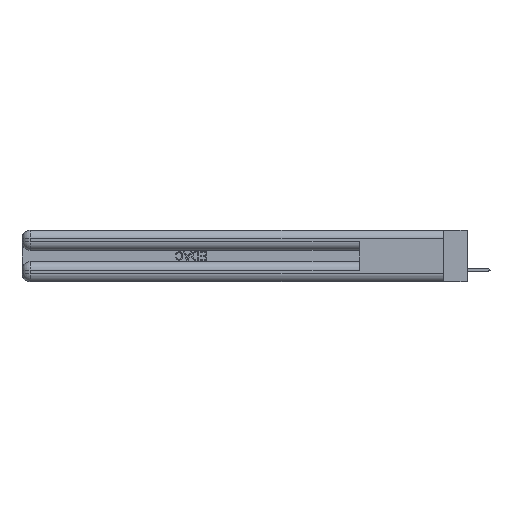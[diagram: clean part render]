
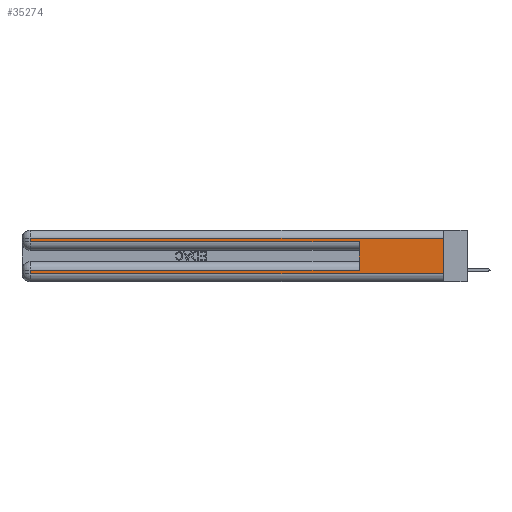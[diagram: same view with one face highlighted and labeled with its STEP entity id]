
A CAD part, left-side view. The second image highlights one B-rep face of the part: STEP entity #35274.
In plain terms, the highlighted planar face has unit normal (-1, 0, 0).
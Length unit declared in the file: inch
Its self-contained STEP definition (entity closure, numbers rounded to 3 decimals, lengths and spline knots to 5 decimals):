
#244 = AXIS2_PLACEMENT_3D ( 'NONE', #25660, #37172, #13451 ) ;
#273 = VECTOR ( 'NONE', #11970, 39.37008 ) ;
#737 = VECTOR ( 'NONE', #44682, 39.37008 ) ;
#2369 = ORIENTED_EDGE ( 'NONE', *, *, #52195, .F. ) ;
#2688 = CARTESIAN_POINT ( 'NONE',  ( 0., 0., 0.06 ) ) ;
#2759 = EDGE_CURVE ( 'NONE', #9822, #37819, #8319, .T. ) ;
#3544 = LINE ( 'NONE', #23982, #273 ) ;
#3567 = ORIENTED_EDGE ( 'NONE', *, *, #43821, .T. ) ;
#4104 = VERTEX_POINT ( 'NONE', #32867 ) ;
#5280 = VECTOR ( 'NONE', #36369, 39.37008 ) ;
#6200 = VERTEX_POINT ( 'NONE', #35007 ) ;
#7194 = DIRECTION ( 'NONE',  ( 0., -1., 0. ) ) ;
#7278 = EDGE_CURVE ( 'NONE', #9822, #4104, #24568, .T. ) ;
#8319 = LINE ( 'NONE', #12839, #49894 ) ;
#9822 = VERTEX_POINT ( 'NONE', #9959 ) ;
#9959 = CARTESIAN_POINT ( 'NONE',  ( 0., 0., 0.31 ) ) ;
#11970 = DIRECTION ( 'NONE',  ( 0., -1., 0. ) ) ;
#12839 = CARTESIAN_POINT ( 'NONE',  ( 0., 0., 0.37 ) ) ;
#13278 = CARTESIAN_POINT ( 'NONE',  ( 0., 2.94, 0.37 ) ) ;
#13451 = DIRECTION ( 'NONE',  ( 0., 0., -1. ) ) ;
#14044 = VERTEX_POINT ( 'NONE', #23625 ) ;
#14071 = EDGE_CURVE ( 'NONE', #27638, #6200, #3544, .T. ) ;
#15268 = EDGE_CURVE ( 'NONE', #44468, #14044, #18999, .T. ) ;
#16174 = CARTESIAN_POINT ( 'NONE',  ( 0., 0.6, 0.145 ) ) ;
#16222 = LINE ( 'NONE', #2688, #24554 ) ;
#18999 = LINE ( 'NONE', #19157, #38222 ) ;
#19157 = CARTESIAN_POINT ( 'NONE',  ( 0., 0., 0.085 ) ) ;
#21005 = DIRECTION ( 'NONE',  ( 0., 0., -1. ) ) ;
#22617 = VECTOR ( 'NONE', #49697, 39.37008 ) ;
#23351 = ORIENTED_EDGE ( 'NONE', *, *, #15268, .T. ) ;
#23366 = VERTEX_POINT ( 'NONE', #47547 ) ;
#23625 = CARTESIAN_POINT ( 'NONE',  ( 0., 2.94, 0.085 ) ) ;
#23982 = CARTESIAN_POINT ( 'NONE',  ( 0., 0., 0.285 ) ) ;
#24554 = VECTOR ( 'NONE', #7194, 39.37008 ) ;
#24568 = LINE ( 'NONE', #24660, #5280 ) ;
#24660 = CARTESIAN_POINT ( 'NONE',  ( 0., 0., 0.31 ) ) ;
#24859 = ORIENTED_EDGE ( 'NONE', *, *, #7278, .T. ) ;
#24878 = CARTESIAN_POINT ( 'NONE',  ( 0., 2.94, 0.37 ) ) ;
#25126 = CARTESIAN_POINT ( 'NONE',  ( 0., 2.94, 0.285 ) ) ;
#25660 = CARTESIAN_POINT ( 'NONE',  ( 0., 0., 0.37 ) ) ;
#26672 = CARTESIAN_POINT ( 'NONE',  ( 0., 0., 0.06 ) ) ;
#26888 = EDGE_CURVE ( 'NONE', #14044, #23366, #27927, .T. ) ;
#27638 = VERTEX_POINT ( 'NONE', #25126 ) ;
#27666 = DIRECTION ( 'NONE',  ( 0., 1., 0. ) ) ;
#27927 = LINE ( 'NONE', #13278, #30411 ) ;
#30411 = VECTOR ( 'NONE', #50302, 39.37008 ) ;
#32867 = CARTESIAN_POINT ( 'NONE',  ( 0., 2.94, 0.31 ) ) ;
#35007 = CARTESIAN_POINT ( 'NONE',  ( 0., 0.6, 0.285 ) ) ;
#35274 = ADVANCED_FACE ( 'NONE', ( #50632 ), #41563, .F. ) ;
#36369 = DIRECTION ( 'NONE',  ( 0., 1., 0. ) ) ;
#37172 = DIRECTION ( 'NONE',  ( 1., 0., 0. ) ) ;
#37363 = LINE ( 'NONE', #16174, #737 ) ;
#37456 = ORIENTED_EDGE ( 'NONE', *, *, #26888, .T. ) ;
#37819 = VERTEX_POINT ( 'NONE', #26672 ) ;
#38222 = VECTOR ( 'NONE', #27666, 39.37008 ) ;
#41563 = PLANE ( 'NONE',  #244 ) ;
#43702 = ORIENTED_EDGE ( 'NONE', *, *, #2759, .F. ) ;
#43821 = EDGE_CURVE ( 'NONE', #4104, #27638, #45172, .T. ) ;
#44468 = VERTEX_POINT ( 'NONE', #48845 ) ;
#44682 = DIRECTION ( 'NONE',  ( 0., 0., 1. ) ) ;
#44870 = ORIENTED_EDGE ( 'NONE', *, *, #14071, .T. ) ;
#45172 = LINE ( 'NONE', #24878, #22617 ) ;
#45265 = EDGE_LOOP ( 'NONE', ( #43702, #24859, #3567, #44870, #2369, #23351, #37456, #48203 ) ) ;
#47547 = CARTESIAN_POINT ( 'NONE',  ( 0., 2.94, 0.06 ) ) ;
#48203 = ORIENTED_EDGE ( 'NONE', *, *, #52606, .T. ) ;
#48845 = CARTESIAN_POINT ( 'NONE',  ( 0., 0.6, 0.085 ) ) ;
#49697 = DIRECTION ( 'NONE',  ( 0., 0., -1. ) ) ;
#49894 = VECTOR ( 'NONE', #21005, 39.37008 ) ;
#50302 = DIRECTION ( 'NONE',  ( 0., 0., -1. ) ) ;
#50632 = FACE_OUTER_BOUND ( 'NONE', #45265, .T. ) ;
#52195 = EDGE_CURVE ( 'NONE', #44468, #6200, #37363, .T. ) ;
#52606 = EDGE_CURVE ( 'NONE', #23366, #37819, #16222, .T. ) ;
